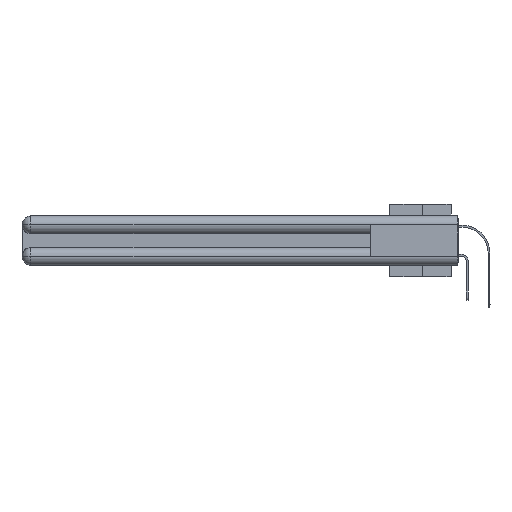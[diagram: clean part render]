
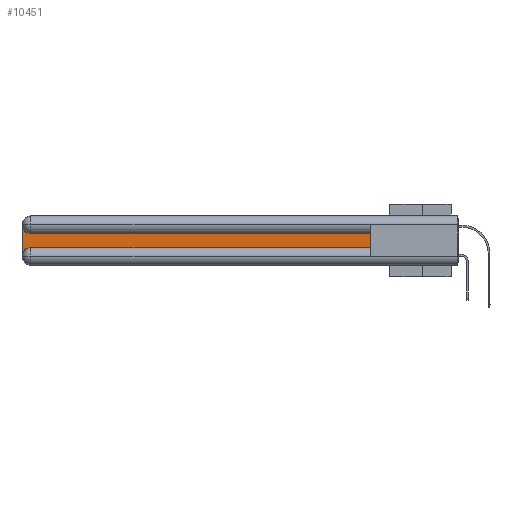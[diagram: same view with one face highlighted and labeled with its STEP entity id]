
A CAD part, left-side view. The second image highlights one B-rep face of the part: STEP entity #10451.
In plain terms, the highlighted planar face has unit normal (-1, 0, 0).
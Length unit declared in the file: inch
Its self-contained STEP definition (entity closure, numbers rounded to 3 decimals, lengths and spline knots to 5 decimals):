
#673 = CARTESIAN_POINT ( 'NONE',  ( 0.075, 0.6, -0.1225 ) ) ;
#1236 = AXIS2_PLACEMENT_3D ( 'NONE', #17620, #8450, #5921 ) ;
#2001 = VERTEX_POINT ( 'NONE', #8813 ) ;
#2353 = VERTEX_POINT ( 'NONE', #4139 ) ;
#3080 = CIRCLE ( 'NONE', #1236, 0.06 ) ;
#3236 = CARTESIAN_POINT ( 'NONE',  ( 0.075, 3., -0.1225 ) ) ;
#3917 = EDGE_CURVE ( 'NONE', #10496, #2353, #5167, .T. ) ;
#4139 = CARTESIAN_POINT ( 'NONE',  ( 0.075, 3., -0.2775 ) ) ;
#5034 = EDGE_CURVE ( 'NONE', #2353, #15265, #15386, .T. ) ;
#5167 = LINE ( 'NONE', #25383, #37672 ) ;
#5751 = CARTESIAN_POINT ( 'NONE',  ( 0.075, 0.6, -0.2175 ) ) ;
#5921 = DIRECTION ( 'NONE',  ( 0., 0., -1. ) ) ;
#6060 = CARTESIAN_POINT ( 'NONE',  ( 0.075, 2.94, -0.2175 ) ) ;
#6204 = VECTOR ( 'NONE', #26922, 39.37008 ) ;
#8450 = DIRECTION ( 'NONE',  ( 1., 0., 0. ) ) ;
#8813 = CARTESIAN_POINT ( 'NONE',  ( 0.075, 2.94, -0.1225 ) ) ;
#9002 = CARTESIAN_POINT ( 'NONE',  ( 0.075, 0.6, -0.1225 ) ) ;
#9277 = DIRECTION ( 'NONE',  ( 0., 0., 1. ) ) ;
#10451 = ADVANCED_FACE ( 'NONE', ( #29866 ), #32975, .F. ) ;
#10496 = VERTEX_POINT ( 'NONE', #30636 ) ;
#11388 = DIRECTION ( 'NONE',  ( 0., 0., -1. ) ) ;
#13375 = DIRECTION ( 'NONE',  ( 0., 0., -1. ) ) ;
#13601 = EDGE_CURVE ( 'NONE', #2001, #10496, #3080, .T. ) ;
#15086 = LINE ( 'NONE', #673, #6204 ) ;
#15265 = VERTEX_POINT ( 'NONE', #6060 ) ;
#15325 = CARTESIAN_POINT ( 'NONE',  ( 0.075, 0.6, -0.2175 ) ) ;
#15386 = CIRCLE ( 'NONE', #37093, 0.06 ) ;
#16864 = AXIS2_PLACEMENT_3D ( 'NONE', #3236, #30248, #18827 ) ;
#17031 = ORIENTED_EDGE ( 'NONE', *, *, #5034, .T. ) ;
#17620 = CARTESIAN_POINT ( 'NONE',  ( 0.075, 2.94, -0.0625 ) ) ;
#18351 = CARTESIAN_POINT ( 'NONE',  ( 0.075, 0.6, -0.2175 ) ) ;
#18827 = DIRECTION ( 'NONE',  ( 0., 0., -1. ) ) ;
#20911 = DIRECTION ( 'NONE',  ( 0., -1., 0. ) ) ;
#22541 = ORIENTED_EDGE ( 'NONE', *, *, #36658, .T. ) ;
#22963 = VECTOR ( 'NONE', #9277, 39.37008 ) ;
#24964 = ORIENTED_EDGE ( 'NONE', *, *, #36998, .T. ) ;
#25383 = CARTESIAN_POINT ( 'NONE',  ( 0.075, 3., -0.2175 ) ) ;
#26175 = LINE ( 'NONE', #5751, #26638 ) ;
#26638 = VECTOR ( 'NONE', #20911, 39.37008 ) ;
#26772 = VERTEX_POINT ( 'NONE', #18351 ) ;
#26922 = DIRECTION ( 'NONE',  ( 0., 1., 0. ) ) ;
#27476 = ORIENTED_EDGE ( 'NONE', *, *, #36086, .T. ) ;
#28484 = VERTEX_POINT ( 'NONE', #9002 ) ;
#29197 = ORIENTED_EDGE ( 'NONE', *, *, #13601, .T. ) ;
#29866 = FACE_OUTER_BOUND ( 'NONE', #34306, .T. ) ;
#30248 = DIRECTION ( 'NONE',  ( 1., 0., 0. ) ) ;
#30636 = CARTESIAN_POINT ( 'NONE',  ( 0.075, 3., -0.0625 ) ) ;
#30840 = ORIENTED_EDGE ( 'NONE', *, *, #3917, .T. ) ;
#30851 = CARTESIAN_POINT ( 'NONE',  ( 0.075, 2.94, -0.2775 ) ) ;
#32975 = PLANE ( 'NONE',  #16864 ) ;
#34306 = EDGE_LOOP ( 'NONE', ( #24964, #29197, #30840, #17031, #27476, #22541 ) ) ;
#35899 = LINE ( 'NONE', #15325, #22963 ) ;
#36086 = EDGE_CURVE ( 'NONE', #15265, #26772, #26175, .T. ) ;
#36474 = DIRECTION ( 'NONE',  ( 1., 0., 0. ) ) ;
#36658 = EDGE_CURVE ( 'NONE', #26772, #28484, #35899, .T. ) ;
#36998 = EDGE_CURVE ( 'NONE', #28484, #2001, #15086, .T. ) ;
#37093 = AXIS2_PLACEMENT_3D ( 'NONE', #30851, #36474, #13375 ) ;
#37672 = VECTOR ( 'NONE', #11388, 39.37008 ) ;
